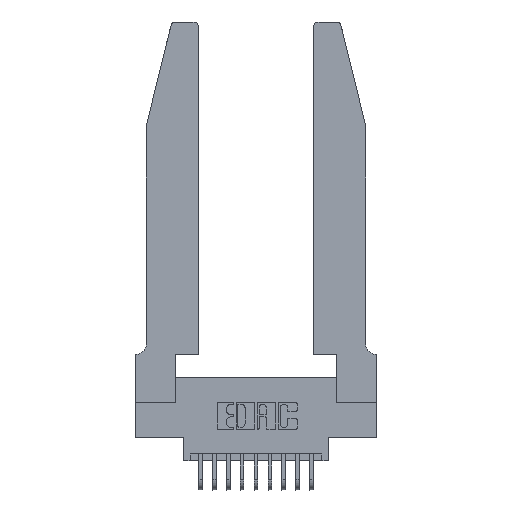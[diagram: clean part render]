
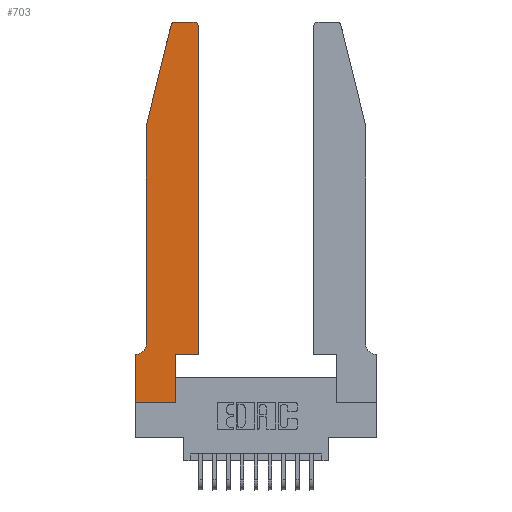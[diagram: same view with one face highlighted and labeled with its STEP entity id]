
A CAD part, top view. The second image highlights one B-rep face of the part: STEP entity #703.
In plain terms, the highlighted planar face has unit normal (0, 0, 1).
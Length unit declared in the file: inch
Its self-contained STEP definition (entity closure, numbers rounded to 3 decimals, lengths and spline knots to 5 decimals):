
#77 = VECTOR ( 'NONE', #15700, 39.37008 ) ;
#95 = CARTESIAN_POINT ( 'NONE',  ( 0.4505, 0.35, 0.37 ) ) ;
#306 = DIRECTION ( 'NONE',  ( 0., 1., 0. ) ) ;
#348 = VECTOR ( 'NONE', #4708, 39.37008 ) ;
#703 = ADVANCED_FACE ( 'NONE', ( #3967 ), #14122, .T. ) ;
#972 = ORIENTED_EDGE ( 'NONE', *, *, #11373, .T. ) ;
#1006 = CARTESIAN_POINT ( 'NONE',  ( 0.4505, 2.72, 0.37 ) ) ;
#1064 = EDGE_CURVE ( 'NONE', #16580, #16320, #9403, .T. ) ;
#1130 = EDGE_CURVE ( 'NONE', #4355, #16580, #11285, .T. ) ;
#1153 = VECTOR ( 'NONE', #15665, 39.37008 ) ;
#1403 = EDGE_CURVE ( 'NONE', #4297, #1626, #15013, .T. ) ;
#1404 = ORIENTED_EDGE ( 'NONE', *, *, #11934, .T. ) ;
#1539 = CARTESIAN_POINT ( 'NONE',  ( 0.284, 2.75, 0.37 ) ) ;
#1626 = VERTEX_POINT ( 'NONE', #8291 ) ;
#1667 = ORIENTED_EDGE ( 'NONE', *, *, #2660, .T. ) ;
#1997 = VERTEX_POINT ( 'NONE', #16493 ) ;
#1998 = LINE ( 'NONE', #3498, #5480 ) ;
#2152 = ORIENTED_EDGE ( 'NONE', *, *, #1403, .T. ) ;
#2433 = AXIS2_PLACEMENT_3D ( 'NONE', #6000, #15394, #7364 ) ;
#2508 = VERTEX_POINT ( 'NONE', #14315 ) ;
#2660 = EDGE_CURVE ( 'NONE', #1626, #4919, #13293, .T. ) ;
#2777 = CIRCLE ( 'NONE', #14790, 0.07 ) ;
#2888 = ORIENTED_EDGE ( 'NONE', *, *, #1130, .T. ) ;
#3198 = VECTOR ( 'NONE', #9263, 39.37008 ) ;
#3417 = ORIENTED_EDGE ( 'NONE', *, *, #1064, .T. ) ;
#3498 = CARTESIAN_POINT ( 'NONE',  ( 0.0755, 2., 0.37 ) ) ;
#3626 = VERTEX_POINT ( 'NONE', #13778 ) ;
#3967 = FACE_OUTER_BOUND ( 'NONE', #4263, .T. ) ;
#4204 = LINE ( 'NONE', #9003, #15050 ) ;
#4263 = EDGE_LOOP ( 'NONE', ( #2888, #3417, #12183, #972, #8768, #8884, #2152, #1667, #15183, #6948, #1404, #9500 ) ) ;
#4297 = VERTEX_POINT ( 'NONE', #18028 ) ;
#4355 = VERTEX_POINT ( 'NONE', #7425 ) ;
#4708 = DIRECTION ( 'NONE',  ( -1., 0., 0. ) ) ;
#4828 = CARTESIAN_POINT ( 'NONE',  ( 0.4505, 0.35, 0.37 ) ) ;
#4919 = VERTEX_POINT ( 'NONE', #8489 ) ;
#5124 = CARTESIAN_POINT ( 'NONE',  ( 0., 0., 0.37 ) ) ;
#5149 = LINE ( 'NONE', #14311, #1153 ) ;
#5307 = CARTESIAN_POINT ( 'NONE',  ( 0., 0., 0.37 ) ) ;
#5480 = VECTOR ( 'NONE', #7788, 39.37008 ) ;
#6000 = CARTESIAN_POINT ( 'NONE',  ( 0.4205, 2.72, 0.37 ) ) ;
#6262 = VERTEX_POINT ( 'NONE', #1006 ) ;
#6665 = AXIS2_PLACEMENT_3D ( 'NONE', #14087, #9612, #9633 ) ;
#6786 = LINE ( 'NONE', #4828, #13508 ) ;
#6948 = ORIENTED_EDGE ( 'NONE', *, *, #14748, .T. ) ;
#7243 = AXIS2_PLACEMENT_3D ( 'NONE', #13553, #13530, #13434 ) ;
#7345 = DIRECTION ( 'NONE',  ( 0., 0., -1. ) ) ;
#7364 = DIRECTION ( 'NONE',  ( 1., 0., 0. ) ) ;
#7425 = CARTESIAN_POINT ( 'NONE',  ( 0.4205, 2.75, 0.37 ) ) ;
#7688 = DIRECTION ( 'NONE',  ( 0., 1., 0. ) ) ;
#7761 = CARTESIAN_POINT ( 'NONE',  ( 0.2605, 2.75, 0.37 ) ) ;
#7788 = DIRECTION ( 'NONE',  ( -0.239, -0.971, 0. ) ) ;
#8016 = VECTOR ( 'NONE', #17984, 39.37008 ) ;
#8114 = CARTESIAN_POINT ( 'NONE',  ( 0.25487, 2.72718, 0.37 ) ) ;
#8291 = CARTESIAN_POINT ( 'NONE',  ( 0., 0., 0.37 ) ) ;
#8489 = CARTESIAN_POINT ( 'NONE',  ( 0.2865, 0., 0.37 ) ) ;
#8768 = ORIENTED_EDGE ( 'NONE', *, *, #14041, .T. ) ;
#8884 = ORIENTED_EDGE ( 'NONE', *, *, #16541, .T. ) ;
#9003 = CARTESIAN_POINT ( 'NONE',  ( 0.4505, 0.35, 0.37 ) ) ;
#9157 = EDGE_CURVE ( 'NONE', #6262, #4355, #13691, .T. ) ;
#9263 = DIRECTION ( 'NONE',  ( 1., 0., 0. ) ) ;
#9403 = CIRCLE ( 'NONE', #7243, 0.03 ) ;
#9500 = ORIENTED_EDGE ( 'NONE', *, *, #9157, .T. ) ;
#9612 = DIRECTION ( 'NONE',  ( 0., 0., 1. ) ) ;
#9633 = DIRECTION ( 'NONE',  ( 1., 0., 0. ) ) ;
#10277 = EDGE_CURVE ( 'NONE', #4919, #11671, #11795, .T. ) ;
#11133 = CARTESIAN_POINT ( 'NONE',  ( 0.2865, 0.35, 0.37 ) ) ;
#11285 = LINE ( 'NONE', #7761, #348 ) ;
#11373 = EDGE_CURVE ( 'NONE', #3626, #1997, #5149, .T. ) ;
#11377 = VECTOR ( 'NONE', #7688, 39.37008 ) ;
#11671 = VERTEX_POINT ( 'NONE', #11133 ) ;
#11795 = LINE ( 'NONE', #15691, #11377 ) ;
#11851 = VERTEX_POINT ( 'NONE', #95 ) ;
#11934 = EDGE_CURVE ( 'NONE', #11851, #6262, #4204, .T. ) ;
#12183 = ORIENTED_EDGE ( 'NONE', *, *, #15282, .T. ) ;
#13293 = LINE ( 'NONE', #5124, #3198 ) ;
#13434 = DIRECTION ( 'NONE',  ( 1., 0., 0. ) ) ;
#13508 = VECTOR ( 'NONE', #15638, 39.37008 ) ;
#13530 = DIRECTION ( 'NONE',  ( 0., 0., 1. ) ) ;
#13553 = CARTESIAN_POINT ( 'NONE',  ( 0.284, 2.72, 0.37 ) ) ;
#13691 = CIRCLE ( 'NONE', #2433, 0.03 ) ;
#13778 = CARTESIAN_POINT ( 'NONE',  ( 0.0755, 2., 0.37 ) ) ;
#14041 = EDGE_CURVE ( 'NONE', #1997, #2508, #2777, .T. ) ;
#14087 = CARTESIAN_POINT ( 'NONE',  ( 0., 0.35, 0.37 ) ) ;
#14122 = PLANE ( 'NONE',  #6665 ) ;
#14311 = CARTESIAN_POINT ( 'NONE',  ( 0.0755, 2., 0.37 ) ) ;
#14315 = CARTESIAN_POINT ( 'NONE',  ( 0.0055, 0.35, 0.37 ) ) ;
#14748 = EDGE_CURVE ( 'NONE', #11671, #11851, #6786, .T. ) ;
#14790 = AXIS2_PLACEMENT_3D ( 'NONE', #15373, #7345, #16713 ) ;
#15013 = LINE ( 'NONE', #5307, #77 ) ;
#15050 = VECTOR ( 'NONE', #306, 39.37008 ) ;
#15120 = LINE ( 'NONE', #17926, #8016 ) ;
#15183 = ORIENTED_EDGE ( 'NONE', *, *, #10277, .T. ) ;
#15282 = EDGE_CURVE ( 'NONE', #16320, #3626, #1998, .T. ) ;
#15373 = CARTESIAN_POINT ( 'NONE',  ( 0.0055, 0.42, 0.37 ) ) ;
#15394 = DIRECTION ( 'NONE',  ( 0., 0., 1. ) ) ;
#15638 = DIRECTION ( 'NONE',  ( 1., 0., 0. ) ) ;
#15665 = DIRECTION ( 'NONE',  ( 0., -1., 0. ) ) ;
#15691 = CARTESIAN_POINT ( 'NONE',  ( 0.2865, 0.35, 0.37 ) ) ;
#15700 = DIRECTION ( 'NONE',  ( 0., -1., 0. ) ) ;
#16320 = VERTEX_POINT ( 'NONE', #8114 ) ;
#16493 = CARTESIAN_POINT ( 'NONE',  ( 0.0755, 0.42, 0.37 ) ) ;
#16541 = EDGE_CURVE ( 'NONE', #2508, #4297, #15120, .T. ) ;
#16580 = VERTEX_POINT ( 'NONE', #1539 ) ;
#16713 = DIRECTION ( 'NONE',  ( -1., 0., 0. ) ) ;
#17926 = CARTESIAN_POINT ( 'NONE',  ( 0.0755, 0.35, 0.37 ) ) ;
#17984 = DIRECTION ( 'NONE',  ( -1., 0., 0. ) ) ;
#18028 = CARTESIAN_POINT ( 'NONE',  ( 0., 0.35, 0.37 ) ) ;
